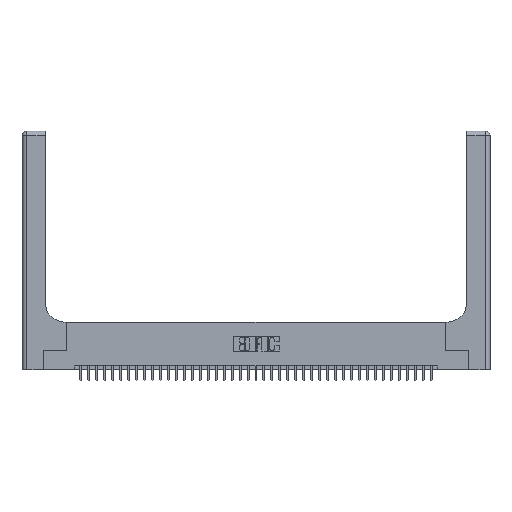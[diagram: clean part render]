
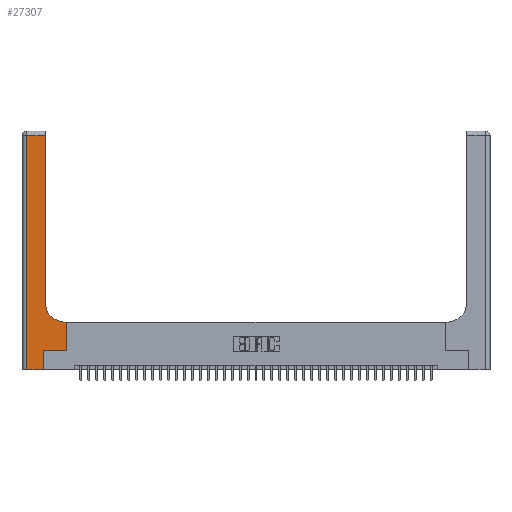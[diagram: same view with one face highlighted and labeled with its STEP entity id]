
A CAD part, top view. The second image highlights one B-rep face of the part: STEP entity #27307.
In plain terms, the highlighted planar face has unit normal (0, 0, 1).
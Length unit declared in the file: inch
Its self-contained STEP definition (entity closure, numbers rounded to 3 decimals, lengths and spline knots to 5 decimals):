
#243 = VECTOR ( 'NONE', #304, 39.37008 ) ;
#304 = DIRECTION ( 'NONE',  ( 1., 0., 0. ) ) ;
#1275 = EDGE_CURVE ( 'NONE', #39944, #10506, #35947, .T. ) ;
#1336 = CARTESIAN_POINT ( 'NONE',  ( 0.06, 2.94, 0.37 ) ) ;
#1578 = CARTESIAN_POINT ( 'NONE',  ( 0.2915, 3., 0.37 ) ) ;
#1804 = VECTOR ( 'NONE', #28103, 39.37008 ) ;
#2659 = FACE_OUTER_BOUND ( 'NONE', #30824, .T. ) ;
#3335 = ORIENTED_EDGE ( 'NONE', *, *, #3989, .T. ) ;
#3374 = LINE ( 'NONE', #10663, #30016 ) ;
#3989 = EDGE_CURVE ( 'NONE', #7028, #23138, #32302, .T. ) ;
#4084 = ORIENTED_EDGE ( 'NONE', *, *, #35602, .T. ) ;
#4495 = DIRECTION ( 'NONE',  ( -1., 0., 0. ) ) ;
#4745 = DIRECTION ( 'NONE',  ( 0., 1., 0. ) ) ;
#4881 = EDGE_CURVE ( 'NONE', #33113, #28629, #17250, .T. ) ;
#5499 = ORIENTED_EDGE ( 'NONE', *, *, #35377, .T. ) ;
#5644 = CARTESIAN_POINT ( 'NONE',  ( 0.2915, 0.6, 0.37 ) ) ;
#6705 = VECTOR ( 'NONE', #4745, 39.37008 ) ;
#7028 = VERTEX_POINT ( 'NONE', #12784 ) ;
#7749 = ORIENTED_EDGE ( 'NONE', *, *, #19264, .T. ) ;
#8491 = VECTOR ( 'NONE', #20375, 39.37008 ) ;
#9321 = EDGE_CURVE ( 'NONE', #21867, #33113, #29512, .T. ) ;
#10411 = DIRECTION ( 'NONE',  ( 0., 1., 0. ) ) ;
#10506 = VERTEX_POINT ( 'NONE', #17809 ) ;
#10663 = CARTESIAN_POINT ( 'NONE',  ( 0., 2.94, 0.37 ) ) ;
#10911 = DIRECTION ( 'NONE',  ( 0., 1., 0. ) ) ;
#11362 = DIRECTION ( 'NONE',  ( 1., 0., 0. ) ) ;
#12222 = ORIENTED_EDGE ( 'NONE', *, *, #1275, .T. ) ;
#12784 = CARTESIAN_POINT ( 'NONE',  ( 0.5585, 0.6, 0.37 ) ) ;
#12848 = CARTESIAN_POINT ( 'NONE',  ( 0.269, 0., 0.37 ) ) ;
#13105 = ORIENTED_EDGE ( 'NONE', *, *, #4881, .T. ) ;
#13405 = CARTESIAN_POINT ( 'NONE',  ( 0., 3., 0.37 ) ) ;
#13966 = AXIS2_PLACEMENT_3D ( 'NONE', #13405, #26291, #4495 ) ;
#13994 = ORIENTED_EDGE ( 'NONE', *, *, #32576, .T. ) ;
#15787 = VECTOR ( 'NONE', #32950, 39.37008 ) ;
#16835 = PLANE ( 'NONE',  #13966 ) ;
#17250 = LINE ( 'NONE', #23659, #15787 ) ;
#17809 = CARTESIAN_POINT ( 'NONE',  ( 0.2915, 2.94, 0.37 ) ) ;
#18153 = VERTEX_POINT ( 'NONE', #22323 ) ;
#18444 = CARTESIAN_POINT ( 'NONE',  ( 0.2915, 0.85, 0.37 ) ) ;
#18779 = CARTESIAN_POINT ( 'NONE',  ( 0., 0., 0.37 ) ) ;
#19264 = EDGE_CURVE ( 'NONE', #18153, #21867, #34636, .T. ) ;
#19464 = VECTOR ( 'NONE', #10911, 39.37008 ) ;
#19493 = DIRECTION ( 'NONE',  ( -1., 0., 0. ) ) ;
#20375 = DIRECTION ( 'NONE',  ( 0., -1., 0. ) ) ;
#21533 = LINE ( 'NONE', #31806, #36048 ) ;
#21867 = VERTEX_POINT ( 'NONE', #12848 ) ;
#22323 = CARTESIAN_POINT ( 'NONE',  ( 0.06, 0., 0.37 ) ) ;
#23100 = ORIENTED_EDGE ( 'NONE', *, *, #26865, .T. ) ;
#23138 = VERTEX_POINT ( 'NONE', #31547 ) ;
#23659 = CARTESIAN_POINT ( 'NONE',  ( 0.269, 0.25, 0.37 ) ) ;
#26291 = DIRECTION ( 'NONE',  ( 0., 0., -1. ) ) ;
#26343 = CARTESIAN_POINT ( 'NONE',  ( 0.5585, 0.25, 0.37 ) ) ;
#26865 = EDGE_CURVE ( 'NONE', #32263, #18153, #40008, .T. ) ;
#27307 = ADVANCED_FACE ( 'NONE', ( #2659 ), #16835, .F. ) ;
#28103 = DIRECTION ( 'NONE',  ( -1., 0., 0. ) ) ;
#28629 = VERTEX_POINT ( 'NONE', #26343 ) ;
#28790 = CARTESIAN_POINT ( 'NONE',  ( 0.269, 0.25, 0.37 ) ) ;
#28977 = ORIENTED_EDGE ( 'NONE', *, *, #9321, .T. ) ;
#29479 = AXIS2_PLACEMENT_3D ( 'NONE', #39257, #33006, #11362 ) ;
#29512 = LINE ( 'NONE', #38887, #6705 ) ;
#30016 = VECTOR ( 'NONE', #19493, 39.37008 ) ;
#30824 = EDGE_LOOP ( 'NONE', ( #12222, #4084, #23100, #7749, #28977, #13105, #13994, #3335, #5499 ) ) ;
#31547 = CARTESIAN_POINT ( 'NONE',  ( 0.5415, 0.6, 0.37 ) ) ;
#31806 = CARTESIAN_POINT ( 'NONE',  ( 0.5585, 0.25, 0.37 ) ) ;
#32263 = VERTEX_POINT ( 'NONE', #1336 ) ;
#32302 = LINE ( 'NONE', #5644, #1804 ) ;
#32576 = EDGE_CURVE ( 'NONE', #28629, #7028, #21533, .T. ) ;
#32950 = DIRECTION ( 'NONE',  ( 1., 0., 0. ) ) ;
#33006 = DIRECTION ( 'NONE',  ( 0., 0., -1. ) ) ;
#33113 = VERTEX_POINT ( 'NONE', #28790 ) ;
#34340 = CIRCLE ( 'NONE', #29479, 0.25 ) ;
#34636 = LINE ( 'NONE', #18779, #243 ) ;
#35377 = EDGE_CURVE ( 'NONE', #23138, #39944, #34340, .T. ) ;
#35566 = CARTESIAN_POINT ( 'NONE',  ( 0.06, 3., 0.37 ) ) ;
#35602 = EDGE_CURVE ( 'NONE', #10506, #32263, #3374, .T. ) ;
#35947 = LINE ( 'NONE', #1578, #19464 ) ;
#36048 = VECTOR ( 'NONE', #10411, 39.37008 ) ;
#38887 = CARTESIAN_POINT ( 'NONE',  ( 0.269, 0., 0.37 ) ) ;
#39257 = CARTESIAN_POINT ( 'NONE',  ( 0.5415, 0.85, 0.37 ) ) ;
#39944 = VERTEX_POINT ( 'NONE', #18444 ) ;
#40008 = LINE ( 'NONE', #35566, #8491 ) ;
